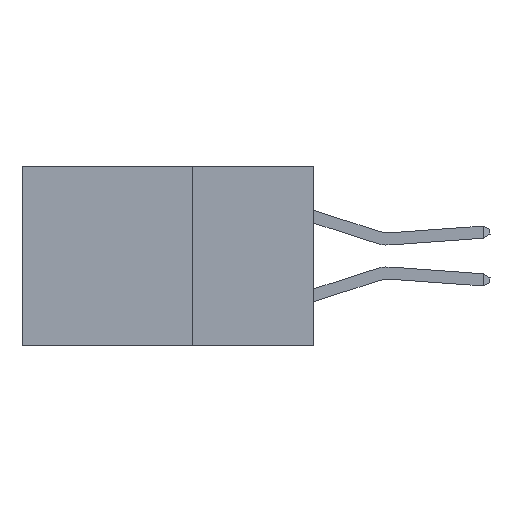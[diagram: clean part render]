
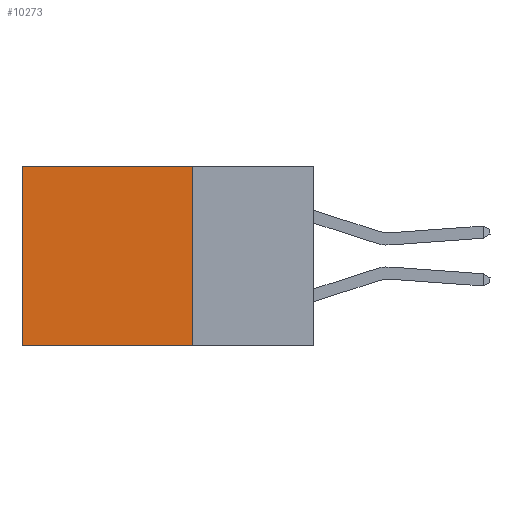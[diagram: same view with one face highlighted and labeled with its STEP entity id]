
A CAD part, left-side view. The second image highlights one B-rep face of the part: STEP entity #10273.
In plain terms, the highlighted planar face has unit normal (-1, 0, 0).
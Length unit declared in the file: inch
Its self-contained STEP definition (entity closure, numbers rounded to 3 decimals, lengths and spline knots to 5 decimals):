
#431 = CARTESIAN_POINT ( 'NONE',  ( 0.2875, 0.25, -0.37 ) ) ;
#1596 = DIRECTION ( 'NONE',  ( 0., 0., -1. ) ) ;
#2183 = DIRECTION ( 'NONE',  ( 0., 1., 0. ) ) ;
#2405 = DIRECTION ( 'NONE',  ( 0., 0., -1. ) ) ;
#4039 = DIRECTION ( 'NONE',  ( 0., 0., -1. ) ) ;
#4758 = CARTESIAN_POINT ( 'NONE',  ( 0.2875, 0.6, 0. ) ) ;
#5436 = LINE ( 'NONE', #10535, #17105 ) ;
#5556 = VECTOR ( 'NONE', #2183, 39.37008 ) ;
#5925 = EDGE_CURVE ( 'NONE', #9358, #19056, #10170, .T. ) ;
#6249 = CARTESIAN_POINT ( 'NONE',  ( 0.2875, 0.25, 0. ) ) ;
#6332 = ORIENTED_EDGE ( 'NONE', *, *, #5925, .F. ) ;
#6448 = VERTEX_POINT ( 'NONE', #8960 ) ;
#7568 = EDGE_CURVE ( 'NONE', #6448, #22425, #12578, .T. ) ;
#7626 = CARTESIAN_POINT ( 'NONE',  ( 0.2875, 0.25, 0. ) ) ;
#7974 = FACE_OUTER_BOUND ( 'NONE', #13416, .T. ) ;
#8960 = CARTESIAN_POINT ( 'NONE',  ( 0.2875, 0.25, 0. ) ) ;
#9080 = PLANE ( 'NONE',  #13072 ) ;
#9158 = DIRECTION ( 'NONE',  ( 1., 0., 0. ) ) ;
#9358 = VERTEX_POINT ( 'NONE', #13865 ) ;
#10170 = LINE ( 'NONE', #431, #5556 ) ;
#10273 = ADVANCED_FACE ( 'NONE', ( #7974 ), #9080, .F. ) ;
#10399 = VECTOR ( 'NONE', #16720, 39.37008 ) ;
#10535 = CARTESIAN_POINT ( 'NONE',  ( 0.2875, 0.6, 0. ) ) ;
#10882 = LINE ( 'NONE', #21485, #11159 ) ;
#11159 = VECTOR ( 'NONE', #2405, 39.37008 ) ;
#11662 = EDGE_CURVE ( 'NONE', #6448, #9358, #10882, .T. ) ;
#11773 = ORIENTED_EDGE ( 'NONE', *, *, #21263, .T. ) ;
#12578 = LINE ( 'NONE', #6249, #10399 ) ;
#13072 = AXIS2_PLACEMENT_3D ( 'NONE', #7626, #9158, #4039 ) ;
#13416 = EDGE_LOOP ( 'NONE', ( #11773, #6332, #13842, #16380 ) ) ;
#13842 = ORIENTED_EDGE ( 'NONE', *, *, #11662, .F. ) ;
#13865 = CARTESIAN_POINT ( 'NONE',  ( 0.2875, 0.25, -0.37 ) ) ;
#16264 = CARTESIAN_POINT ( 'NONE',  ( 0.2875, 0.6, -0.37 ) ) ;
#16380 = ORIENTED_EDGE ( 'NONE', *, *, #7568, .T. ) ;
#16720 = DIRECTION ( 'NONE',  ( 0., 1., 0. ) ) ;
#17105 = VECTOR ( 'NONE', #1596, 39.37008 ) ;
#19056 = VERTEX_POINT ( 'NONE', #16264 ) ;
#21263 = EDGE_CURVE ( 'NONE', #22425, #19056, #5436, .T. ) ;
#21485 = CARTESIAN_POINT ( 'NONE',  ( 0.2875, 0.25, 0. ) ) ;
#22425 = VERTEX_POINT ( 'NONE', #4758 ) ;
